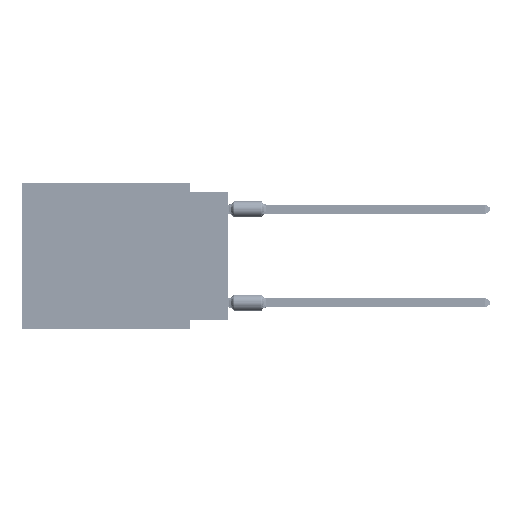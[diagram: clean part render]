
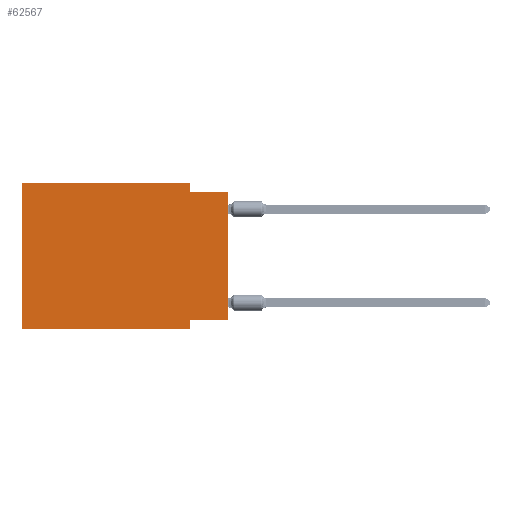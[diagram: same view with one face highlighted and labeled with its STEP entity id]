
A CAD part, left-side view. The second image highlights one B-rep face of the part: STEP entity #62567.
In plain terms, the highlighted planar face has unit normal (-1, 0, 0).
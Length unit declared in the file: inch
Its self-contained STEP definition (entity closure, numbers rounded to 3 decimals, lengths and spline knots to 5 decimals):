
#20 = LINE ( 'NONE', #52686, #7507 ) ;
#96 = DIRECTION ( 'NONE',  ( 0., 0., -1. ) ) ;
#373 = ORIENTED_EDGE ( 'NONE', *, *, #53532, .F. ) ;
#762 = PLANE ( 'NONE',  #27181 ) ;
#1073 = VECTOR ( 'NONE', #24737, 39.37008 ) ;
#2846 = VERTEX_POINT ( 'NONE', #14610 ) ;
#3099 = LINE ( 'NONE', #60920, #21987 ) ;
#5218 = CARTESIAN_POINT ( 'NONE',  ( 0., 0.55, 0. ) ) ;
#6482 = ORIENTED_EDGE ( 'NONE', *, *, #33665, .T. ) ;
#7507 = VECTOR ( 'NONE', #26993, 39.37008 ) ;
#7771 = ORIENTED_EDGE ( 'NONE', *, *, #31023, .F. ) ;
#8442 = VERTEX_POINT ( 'NONE', #20284 ) ;
#9069 = LINE ( 'NONE', #67600, #16801 ) ;
#11692 = VERTEX_POINT ( 'NONE', #43374 ) ;
#13481 = CARTESIAN_POINT ( 'NONE',  ( 0., 0.1, 0. ) ) ;
#14255 = VECTOR ( 'NONE', #58281, 39.37008 ) ;
#14610 = CARTESIAN_POINT ( 'NONE',  ( 0., 0.1, -0.365 ) ) ;
#15093 = ORIENTED_EDGE ( 'NONE', *, *, #29364, .T. ) ;
#15538 = VECTOR ( 'NONE', #21083, 39.37008 ) ;
#16193 = CARTESIAN_POINT ( 'NONE',  ( 0., 0., -0.365 ) ) ;
#16801 = VECTOR ( 'NONE', #25124, 39.37008 ) ;
#18590 = LINE ( 'NONE', #13481, #26983 ) ;
#19759 = ORIENTED_EDGE ( 'NONE', *, *, #53533, .F. ) ;
#20284 = CARTESIAN_POINT ( 'NONE',  ( 0., 0.55, 0. ) ) ;
#20601 = ORIENTED_EDGE ( 'NONE', *, *, #45269, .F. ) ;
#21083 = DIRECTION ( 'NONE',  ( 0., -1., 0. ) ) ;
#21987 = VECTOR ( 'NONE', #32283, 39.37008 ) ;
#24225 = ORIENTED_EDGE ( 'NONE', *, *, #64167, .F. ) ;
#24737 = DIRECTION ( 'NONE',  ( 0., -1., 0. ) ) ;
#25124 = DIRECTION ( 'NONE',  ( 0., 1., 0. ) ) ;
#25543 = CARTESIAN_POINT ( 'NONE',  ( 0., 0.55, -0.39 ) ) ;
#26057 = DIRECTION ( 'NONE',  ( 1., 0., 0. ) ) ;
#26983 = VECTOR ( 'NONE', #53899, 39.37008 ) ;
#26993 = DIRECTION ( 'NONE',  ( 0., -1., 0. ) ) ;
#27107 = CARTESIAN_POINT ( 'NONE',  ( 0., 0.55, 0. ) ) ;
#27181 = AXIS2_PLACEMENT_3D ( 'NONE', #5218, #26057, #96 ) ;
#28733 = VERTEX_POINT ( 'NONE', #16193 ) ;
#29364 = EDGE_CURVE ( 'NONE', #11692, #44372, #40953, .T. ) ;
#29596 = VECTOR ( 'NONE', #53467, 39.37008 ) ;
#29897 = LINE ( 'NONE', #30568, #1073 ) ;
#30568 = CARTESIAN_POINT ( 'NONE',  ( 0., 0., -0.025 ) ) ;
#31023 = EDGE_CURVE ( 'NONE', #28733, #2846, #9069, .T. ) ;
#32258 = LINE ( 'NONE', #27107, #29596 ) ;
#32283 = DIRECTION ( 'NONE',  ( 0., 0., 1. ) ) ;
#33665 = EDGE_CURVE ( 'NONE', #28733, #35059, #3099, .T. ) ;
#35059 = VERTEX_POINT ( 'NONE', #61010 ) ;
#35603 = CARTESIAN_POINT ( 'NONE',  ( 0., 0.1, -0.39 ) ) ;
#40953 = LINE ( 'NONE', #25543, #15538 ) ;
#42080 = EDGE_CURVE ( 'NONE', #58309, #47113, #18590, .T. ) ;
#43327 = CARTESIAN_POINT ( 'NONE',  ( 0., 0.1, 0. ) ) ;
#43374 = CARTESIAN_POINT ( 'NONE',  ( 0., 0.55, -0.39 ) ) ;
#44372 = VERTEX_POINT ( 'NONE', #35603 ) ;
#45269 = EDGE_CURVE ( 'NONE', #47113, #35059, #29897, .T. ) ;
#47113 = VERTEX_POINT ( 'NONE', #66762 ) ;
#47612 = FACE_OUTER_BOUND ( 'NONE', #57579, .T. ) ;
#48665 = LINE ( 'NONE', #53138, #14255 ) ;
#50700 = ORIENTED_EDGE ( 'NONE', *, *, #42080, .F. ) ;
#52686 = CARTESIAN_POINT ( 'NONE',  ( 0., 0.55, 0. ) ) ;
#53138 = CARTESIAN_POINT ( 'NONE',  ( 0., 0.1, -0.39 ) ) ;
#53467 = DIRECTION ( 'NONE',  ( 0., 0., 1. ) ) ;
#53532 = EDGE_CURVE ( 'NONE', #11692, #8442, #32258, .T. ) ;
#53533 = EDGE_CURVE ( 'NONE', #2846, #44372, #48665, .T. ) ;
#53899 = DIRECTION ( 'NONE',  ( 0., 0., -1. ) ) ;
#57579 = EDGE_LOOP ( 'NONE', ( #6482, #20601, #50700, #24225, #373, #15093, #19759, #7771 ) ) ;
#58281 = DIRECTION ( 'NONE',  ( 0., 0., -1. ) ) ;
#58309 = VERTEX_POINT ( 'NONE', #43327 ) ;
#60920 = CARTESIAN_POINT ( 'NONE',  ( 0., 0., 0. ) ) ;
#61010 = CARTESIAN_POINT ( 'NONE',  ( 0., 0., -0.025 ) ) ;
#62567 = ADVANCED_FACE ( 'NONE', ( #47612 ), #762, .F. ) ;
#64167 = EDGE_CURVE ( 'NONE', #8442, #58309, #20, .T. ) ;
#66762 = CARTESIAN_POINT ( 'NONE',  ( 0., 0.1, -0.025 ) ) ;
#67600 = CARTESIAN_POINT ( 'NONE',  ( 0., 0., -0.365 ) ) ;
